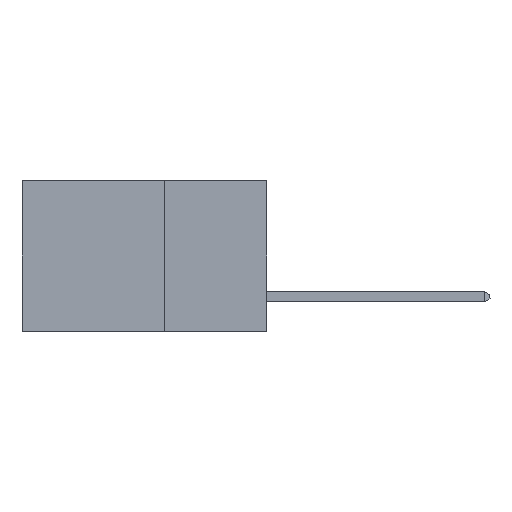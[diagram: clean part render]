
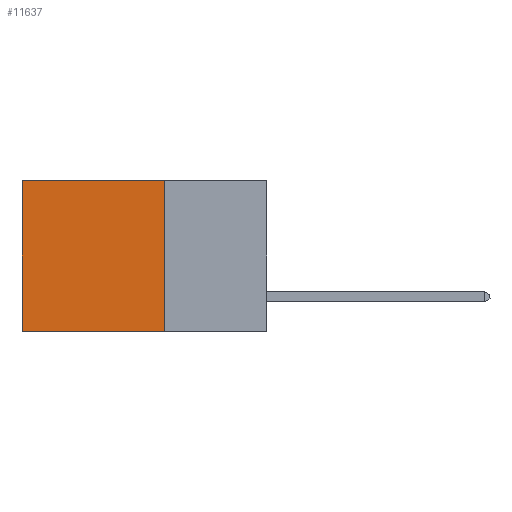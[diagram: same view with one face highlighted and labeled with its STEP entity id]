
A CAD part, left-side view. The second image highlights one B-rep face of the part: STEP entity #11637.
In plain terms, the highlighted planar face has unit normal (-1, 0, 0).
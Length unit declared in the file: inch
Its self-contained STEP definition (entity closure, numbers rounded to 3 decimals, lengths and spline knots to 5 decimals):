
#2706 = VECTOR ( 'NONE', #24345, 39.37008 ) ;
#2872 = CARTESIAN_POINT ( 'NONE',  ( 0.2875, 0.25, -0.37 ) ) ;
#4580 = AXIS2_PLACEMENT_3D ( 'NONE', #15558, #26037, #13557 ) ;
#5137 = VERTEX_POINT ( 'NONE', #23644 ) ;
#5154 = VERTEX_POINT ( 'NONE', #17545 ) ;
#5308 = EDGE_CURVE ( 'NONE', #7764, #5137, #17299, .T. ) ;
#7130 = VECTOR ( 'NONE', #16396, 39.37008 ) ;
#7213 = PLANE ( 'NONE',  #4580 ) ;
#7764 = VERTEX_POINT ( 'NONE', #25036 ) ;
#8070 = CARTESIAN_POINT ( 'NONE',  ( 0.2875, 0.6, 0. ) ) ;
#9159 = EDGE_LOOP ( 'NONE', ( #23490, #20227, #23828, #12417 ) ) ;
#9358 = EDGE_CURVE ( 'NONE', #7764, #5154, #14003, .T. ) ;
#10775 = LINE ( 'NONE', #8070, #7130 ) ;
#11637 = ADVANCED_FACE ( 'NONE', ( #22634 ), #7213, .F. ) ;
#11869 = CARTESIAN_POINT ( 'NONE',  ( 0.2875, 0.25, 0. ) ) ;
#12417 = ORIENTED_EDGE ( 'NONE', *, *, #5308, .T. ) ;
#12451 = VECTOR ( 'NONE', #22090, 39.37008 ) ;
#13557 = DIRECTION ( 'NONE',  ( 0., 0., -1. ) ) ;
#13818 = CARTESIAN_POINT ( 'NONE',  ( 0.2875, 0.25, 0. ) ) ;
#14003 = LINE ( 'NONE', #11869, #2706 ) ;
#15558 = CARTESIAN_POINT ( 'NONE',  ( 0.2875, 0.25, 0. ) ) ;
#16396 = DIRECTION ( 'NONE',  ( 0., 0., -1. ) ) ;
#16468 = VERTEX_POINT ( 'NONE', #24000 ) ;
#17299 = LINE ( 'NONE', #13818, #12451 ) ;
#17545 = CARTESIAN_POINT ( 'NONE',  ( 0.2875, 0.25, -0.37 ) ) ;
#17635 = DIRECTION ( 'NONE',  ( 0., 1., 0. ) ) ;
#20227 = ORIENTED_EDGE ( 'NONE', *, *, #26009, .F. ) ;
#22090 = DIRECTION ( 'NONE',  ( 0., 1., 0. ) ) ;
#22634 = FACE_OUTER_BOUND ( 'NONE', #9159, .T. ) ;
#23490 = ORIENTED_EDGE ( 'NONE', *, *, #23852, .T. ) ;
#23644 = CARTESIAN_POINT ( 'NONE',  ( 0.2875, 0.6, 0. ) ) ;
#23828 = ORIENTED_EDGE ( 'NONE', *, *, #9358, .F. ) ;
#23852 = EDGE_CURVE ( 'NONE', #5137, #16468, #10775, .T. ) ;
#24000 = CARTESIAN_POINT ( 'NONE',  ( 0.2875, 0.6, -0.37 ) ) ;
#24345 = DIRECTION ( 'NONE',  ( 0., 0., -1. ) ) ;
#25036 = CARTESIAN_POINT ( 'NONE',  ( 0.2875, 0.25, 0. ) ) ;
#25956 = LINE ( 'NONE', #2872, #26595 ) ;
#26009 = EDGE_CURVE ( 'NONE', #5154, #16468, #25956, .T. ) ;
#26037 = DIRECTION ( 'NONE',  ( 1., 0., 0. ) ) ;
#26595 = VECTOR ( 'NONE', #17635, 39.37008 ) ;
